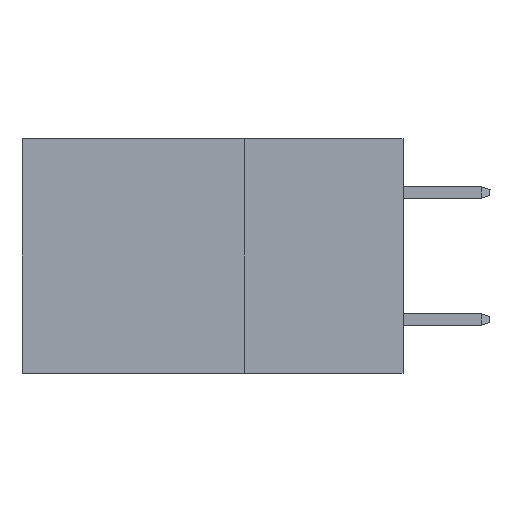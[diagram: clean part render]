
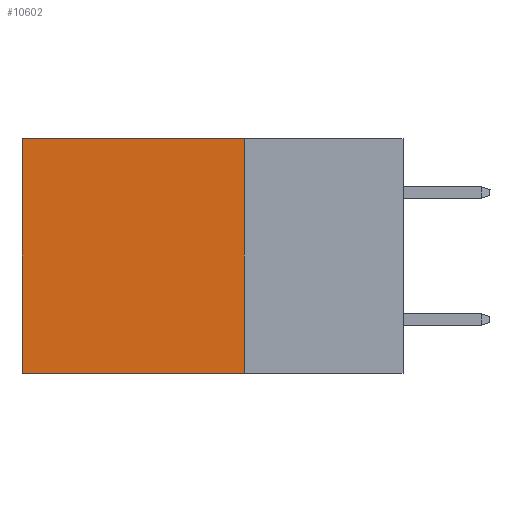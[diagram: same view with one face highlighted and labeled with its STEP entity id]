
A CAD part, left-side view. The second image highlights one B-rep face of the part: STEP entity #10602.
In plain terms, the highlighted planar face has unit normal (-1, 0, 0).
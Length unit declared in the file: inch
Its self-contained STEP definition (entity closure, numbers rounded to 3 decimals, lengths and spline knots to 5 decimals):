
#84 = DIRECTION ( 'NONE',  ( 1., 0., 0. ) ) ;
#740 = VECTOR ( 'NONE', #5283, 39.37008 ) ;
#819 = DIRECTION ( 'NONE',  ( 0., 0., -1. ) ) ;
#2345 = CARTESIAN_POINT ( 'NONE',  ( 0.2875, 0.25, -0.37 ) ) ;
#2531 = LINE ( 'NONE', #7443, #3515 ) ;
#2955 = CARTESIAN_POINT ( 'NONE',  ( 0.2875, 0.25, 0. ) ) ;
#3515 = VECTOR ( 'NONE', #24570, 39.37008 ) ;
#5026 = EDGE_CURVE ( 'NONE', #23142, #11057, #11605, .T. ) ;
#5283 = DIRECTION ( 'NONE',  ( 0., 0., -1. ) ) ;
#7002 = CARTESIAN_POINT ( 'NONE',  ( 0.2875, 0.6, -0.37 ) ) ;
#7443 = CARTESIAN_POINT ( 'NONE',  ( 0.2875, 0.25, 0. ) ) ;
#8021 = CARTESIAN_POINT ( 'NONE',  ( 0.2875, 0.6, 0. ) ) ;
#8990 = VERTEX_POINT ( 'NONE', #10426 ) ;
#10426 = CARTESIAN_POINT ( 'NONE',  ( 0.2875, 0.6, 0. ) ) ;
#10602 = ADVANCED_FACE ( 'NONE', ( #23870 ), #11040, .F. ) ;
#11040 = PLANE ( 'NONE',  #18148 ) ;
#11057 = VERTEX_POINT ( 'NONE', #15723 ) ;
#11256 = ORIENTED_EDGE ( 'NONE', *, *, #12411, .F. ) ;
#11605 = LINE ( 'NONE', #2955, #14110 ) ;
#12403 = CARTESIAN_POINT ( 'NONE',  ( 0.2875, 0.25, 0. ) ) ;
#12411 = EDGE_CURVE ( 'NONE', #11057, #26304, #13313, .T. ) ;
#13313 = LINE ( 'NONE', #2345, #21968 ) ;
#13338 = DIRECTION ( 'NONE',  ( 0., 0., -1. ) ) ;
#14110 = VECTOR ( 'NONE', #819, 39.37008 ) ;
#15337 = ORIENTED_EDGE ( 'NONE', *, *, #23584, .T. ) ;
#15723 = CARTESIAN_POINT ( 'NONE',  ( 0.2875, 0.25, -0.37 ) ) ;
#16280 = ORIENTED_EDGE ( 'NONE', *, *, #21092, .T. ) ;
#17094 = ORIENTED_EDGE ( 'NONE', *, *, #5026, .F. ) ;
#18148 = AXIS2_PLACEMENT_3D ( 'NONE', #19388, #84, #13338 ) ;
#19388 = CARTESIAN_POINT ( 'NONE',  ( 0.2875, 0.25, 0. ) ) ;
#21092 = EDGE_CURVE ( 'NONE', #23142, #8990, #2531, .T. ) ;
#21968 = VECTOR ( 'NONE', #28114, 39.37008 ) ;
#22145 = EDGE_LOOP ( 'NONE', ( #15337, #11256, #17094, #16280 ) ) ;
#23142 = VERTEX_POINT ( 'NONE', #12403 ) ;
#23584 = EDGE_CURVE ( 'NONE', #8990, #26304, #25020, .T. ) ;
#23870 = FACE_OUTER_BOUND ( 'NONE', #22145, .T. ) ;
#24570 = DIRECTION ( 'NONE',  ( 0., 1., 0. ) ) ;
#25020 = LINE ( 'NONE', #8021, #740 ) ;
#26304 = VERTEX_POINT ( 'NONE', #7002 ) ;
#28114 = DIRECTION ( 'NONE',  ( 0., 1., 0. ) ) ;
